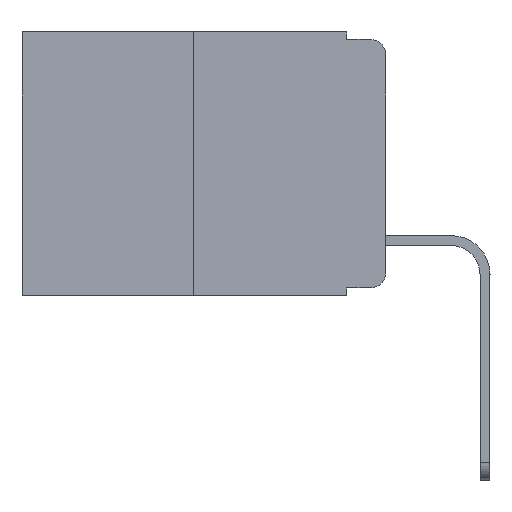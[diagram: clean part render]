
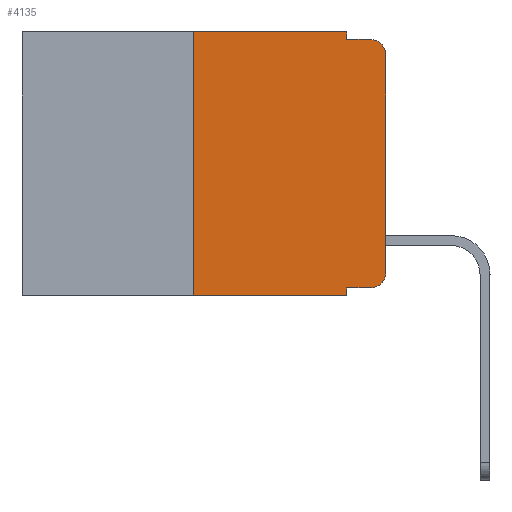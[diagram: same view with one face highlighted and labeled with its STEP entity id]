
A CAD part, left-side view. The second image highlights one B-rep face of the part: STEP entity #4135.
In plain terms, the highlighted planar face has unit normal (-1, 0, 0).
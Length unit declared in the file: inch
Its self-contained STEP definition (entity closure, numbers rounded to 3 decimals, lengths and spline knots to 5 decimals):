
#217 = DIRECTION ( 'NONE',  ( 0., 0., 1. ) ) ;
#252 = CARTESIAN_POINT ( 'NONE',  ( 0., 0., 0. ) ) ;
#262 = LINE ( 'NONE', #11440, #6823 ) ;
#263 = CARTESIAN_POINT ( 'NONE',  ( 0., 0., -0.313 ) ) ;
#331 = EDGE_CURVE ( 'NONE', #8159, #7293, #6954, .T. ) ;
#358 = CARTESIAN_POINT ( 'NONE',  ( 0., 0.25, 0. ) ) ;
#377 = VERTEX_POINT ( 'NONE', #6075 ) ;
#548 = VECTOR ( 'NONE', #217, 39.37008 ) ;
#743 = LINE ( 'NONE', #2614, #5373 ) ;
#811 = ORIENTED_EDGE ( 'NONE', *, *, #1178, .T. ) ;
#1001 = LINE ( 'NONE', #7612, #2401 ) ;
#1166 = ORIENTED_EDGE ( 'NONE', *, *, #331, .F. ) ;
#1178 = EDGE_CURVE ( 'NONE', #7032, #6895, #10609, .T. ) ;
#1457 = LINE ( 'NONE', #358, #8457 ) ;
#1475 = CARTESIAN_POINT ( 'NONE',  ( 0., 0.473, 0. ) ) ;
#1597 = DIRECTION ( 'NONE',  ( 0., -1., 0. ) ) ;
#1729 = VECTOR ( 'NONE', #8802, 39.37008 ) ;
#1825 = CARTESIAN_POINT ( 'NONE',  ( 0., 0.02, -0.313 ) ) ;
#2050 = AXIS2_PLACEMENT_3D ( 'NONE', #1825, #2812, #3709 ) ;
#2291 = VECTOR ( 'NONE', #9602, 39.37008 ) ;
#2401 = VECTOR ( 'NONE', #5847, 39.37008 ) ;
#2614 = CARTESIAN_POINT ( 'NONE',  ( 0., 0.051, 0. ) ) ;
#2745 = VERTEX_POINT ( 'NONE', #7376 ) ;
#2812 = DIRECTION ( 'NONE',  ( -1., 0., 0. ) ) ;
#2943 = EDGE_CURVE ( 'NONE', #10683, #6895, #7878, .T. ) ;
#3053 = EDGE_CURVE ( 'NONE', #377, #10683, #743, .T. ) ;
#3341 = CARTESIAN_POINT ( 'NONE',  ( 0., 0.473, 0. ) ) ;
#3387 = PLANE ( 'NONE',  #8956 ) ;
#3709 = DIRECTION ( 'NONE',  ( 0., 0., -1. ) ) ;
#3827 = ORIENTED_EDGE ( 'NONE', *, *, #3053, .F. ) ;
#3891 = CARTESIAN_POINT ( 'NONE',  ( 0., 0.051, -0.343 ) ) ;
#4080 = CARTESIAN_POINT ( 'NONE',  ( 0., 0.25, -0.343 ) ) ;
#4100 = ORIENTED_EDGE ( 'NONE', *, *, #7470, .T. ) ;
#4135 = ADVANCED_FACE ( 'NONE', ( #8563 ), #3387, .F. ) ;
#4998 = CARTESIAN_POINT ( 'NONE',  ( 0., 0.051, 0. ) ) ;
#5006 = EDGE_CURVE ( 'NONE', #7272, #7032, #10646, .T. ) ;
#5066 = CIRCLE ( 'NONE', #2050, 0.02 ) ;
#5146 = VECTOR ( 'NONE', #5892, 39.37008 ) ;
#5220 = ORIENTED_EDGE ( 'NONE', *, *, #7632, .T. ) ;
#5316 = DIRECTION ( 'NONE',  ( 0., 0., -1. ) ) ;
#5359 = DIRECTION ( 'NONE',  ( -1., 0., 0. ) ) ;
#5373 = VECTOR ( 'NONE', #5316, 39.37008 ) ;
#5479 = EDGE_CURVE ( 'NONE', #10914, #7293, #262, .T. ) ;
#5757 = ORIENTED_EDGE ( 'NONE', *, *, #5933, .F. ) ;
#5847 = DIRECTION ( 'NONE',  ( 0., -1., 0. ) ) ;
#5892 = DIRECTION ( 'NONE',  ( 0., 0., -1. ) ) ;
#5933 = EDGE_CURVE ( 'NONE', #8436, #377, #11418, .T. ) ;
#5971 = CARTESIAN_POINT ( 'NONE',  ( 0., 0.051, -0.01 ) ) ;
#6008 = DIRECTION ( 'NONE',  ( 0., 0., -1. ) ) ;
#6075 = CARTESIAN_POINT ( 'NONE',  ( 0., 0.051, 0. ) ) ;
#6341 = EDGE_CURVE ( 'NONE', #10914, #8436, #1457, .T. ) ;
#6443 = ORIENTED_EDGE ( 'NONE', *, *, #5006, .T. ) ;
#6823 = VECTOR ( 'NONE', #1597, 39.37008 ) ;
#6895 = VERTEX_POINT ( 'NONE', #8857 ) ;
#6954 = LINE ( 'NONE', #4998, #5146 ) ;
#7032 = VERTEX_POINT ( 'NONE', #7432 ) ;
#7272 = VERTEX_POINT ( 'NONE', #263 ) ;
#7293 = VERTEX_POINT ( 'NONE', #3891 ) ;
#7307 = CARTESIAN_POINT ( 'NONE',  ( 0., 0.02, -0.03 ) ) ;
#7376 = CARTESIAN_POINT ( 'NONE',  ( 0., 0.02, -0.333 ) ) ;
#7432 = CARTESIAN_POINT ( 'NONE',  ( 0., 0., -0.03 ) ) ;
#7470 = EDGE_CURVE ( 'NONE', #8159, #2745, #1001, .T. ) ;
#7612 = CARTESIAN_POINT ( 'NONE',  ( 0., 0.051, -0.333 ) ) ;
#7632 = EDGE_CURVE ( 'NONE', #2745, #7272, #5066, .T. ) ;
#7878 = LINE ( 'NONE', #5971, #2291 ) ;
#8159 = VERTEX_POINT ( 'NONE', #9598 ) ;
#8171 = DIRECTION ( 'NONE',  ( 0., 0., -1. ) ) ;
#8436 = VERTEX_POINT ( 'NONE', #11079 ) ;
#8457 = VECTOR ( 'NONE', #9469, 39.37008 ) ;
#8563 = FACE_OUTER_BOUND ( 'NONE', #9476, .T. ) ;
#8802 = DIRECTION ( 'NONE',  ( 0., -1., 0. ) ) ;
#8857 = CARTESIAN_POINT ( 'NONE',  ( 0., 0.02, -0.01 ) ) ;
#8956 = AXIS2_PLACEMENT_3D ( 'NONE', #1475, #11392, #6008 ) ;
#9301 = ORIENTED_EDGE ( 'NONE', *, *, #5479, .T. ) ;
#9469 = DIRECTION ( 'NONE',  ( 0., 0., 1. ) ) ;
#9476 = EDGE_LOOP ( 'NONE', ( #6443, #811, #10165, #3827, #5757, #9615, #9301, #1166, #4100, #5220 ) ) ;
#9598 = CARTESIAN_POINT ( 'NONE',  ( 0., 0.051, -0.333 ) ) ;
#9602 = DIRECTION ( 'NONE',  ( 0., -1., 0. ) ) ;
#9615 = ORIENTED_EDGE ( 'NONE', *, *, #6341, .F. ) ;
#10165 = ORIENTED_EDGE ( 'NONE', *, *, #2943, .F. ) ;
#10609 = CIRCLE ( 'NONE', #11574, 0.02 ) ;
#10646 = LINE ( 'NONE', #252, #548 ) ;
#10683 = VERTEX_POINT ( 'NONE', #10821 ) ;
#10821 = CARTESIAN_POINT ( 'NONE',  ( 0., 0.051, -0.01 ) ) ;
#10914 = VERTEX_POINT ( 'NONE', #4080 ) ;
#11079 = CARTESIAN_POINT ( 'NONE',  ( 0., 0.25, 0. ) ) ;
#11392 = DIRECTION ( 'NONE',  ( 1., 0., 0. ) ) ;
#11418 = LINE ( 'NONE', #3341, #1729 ) ;
#11440 = CARTESIAN_POINT ( 'NONE',  ( 0., 0.473, -0.343 ) ) ;
#11574 = AXIS2_PLACEMENT_3D ( 'NONE', #7307, #5359, #8171 ) ;
